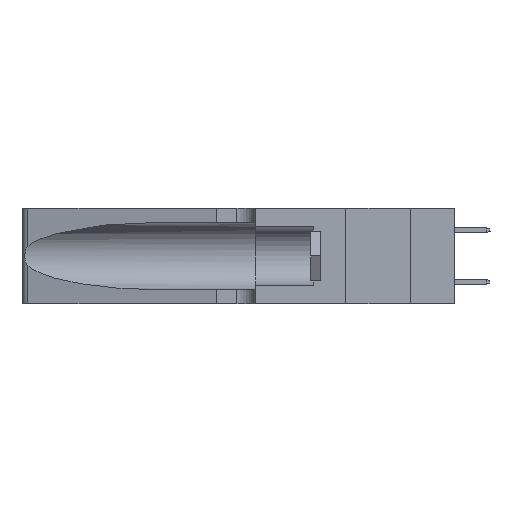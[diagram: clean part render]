
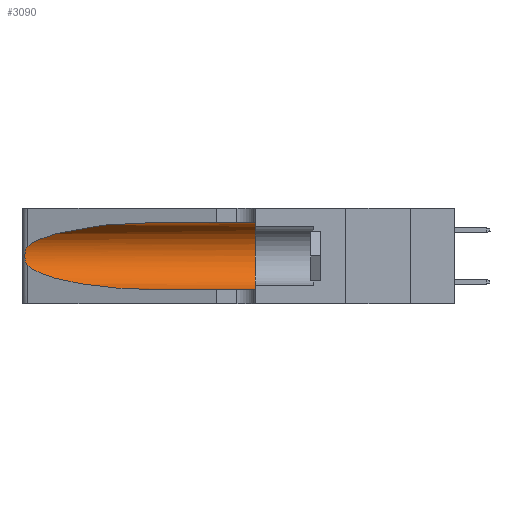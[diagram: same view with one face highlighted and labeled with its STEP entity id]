
A CAD part, left-side view. The second image highlights one B-rep face of the part: STEP entity #3090.
In plain terms, the highlighted cylindrical face has radius 3.308 mm (diameter 6.617 mm), a partial arc.
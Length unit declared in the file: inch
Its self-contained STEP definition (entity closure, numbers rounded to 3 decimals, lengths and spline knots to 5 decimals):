
#800 = VERTEX_POINT ( 'NONE', #20924 ) ;
#1029 = CARTESIAN_POINT ( 'NONE',  ( 0.25555, 1.22994, 0.2215 ) ) ;
#1853 = LINE ( 'NONE', #12380, #35251 ) ;
#2455 = EDGE_CURVE ( 'NONE', #5879, #4139, #14747, .T. ) ;
#2764 = EDGE_CURVE ( 'NONE', #34882, #5879, #6624, .T. ) ;
#3090 = ADVANCED_FACE ( 'NONE', ( #40278 ), #20788, .F. ) ;
#3096 = ORIENTED_EDGE ( 'NONE', *, *, #25256, .F. ) ;
#3694 = CARTESIAN_POINT ( 'NONE',  ( 0.25555, 1.22993, 0.14849 ) ) ;
#3937 = CARTESIAN_POINT ( 'NONE',  ( 0.25487, 1.22718, 0.22369 ) ) ;
#4139 = VERTEX_POINT ( 'NONE', #7296 ) ;
#5879 = VERTEX_POINT ( 'NONE', #3937 ) ;
#6624 =( BOUNDED_CURVE ( )  B_SPLINE_CURVE ( 3, ( #34306, #25080, #31236, #22221 ),
 .UNSPECIFIED., .F., .F. ) 
 B_SPLINE_CURVE_WITH_KNOTS ( ( 4, 4 ),
 ( 1.5708, 2.84003 ),
 .UNSPECIFIED. ) 
 CURVE ( )  GEOMETRIC_REPRESENTATION_ITEM ( )  RATIONAL_B_SPLINE_CURVE ( ( 1., 0.87, 0.87, 1. ) ) 
 REPRESENTATION_ITEM ( '' )  );
#7296 = CARTESIAN_POINT ( 'NONE',  ( 0.25487, 1.22718, 0.14631 ) ) ;
#7967 =( BOUNDED_CURVE ( )  B_SPLINE_CURVE ( 3, ( #25918, #32053, #32248, #25720 ),
 .UNSPECIFIED., .F., .F. ) 
 B_SPLINE_CURVE_WITH_KNOTS ( ( 4, 4 ),
 ( 3.44316, 4.71239 ),
 .UNSPECIFIED. ) 
 CURVE ( )  GEOMETRIC_REPRESENTATION_ITEM ( )  RATIONAL_B_SPLINE_CURVE ( ( 1., 0.87, 0.87, 1. ) ) 
 REPRESENTATION_ITEM ( '' )  );
#8767 = ORIENTED_EDGE ( 'NONE', *, *, #2455, .T. ) ;
#9604 = AXIS2_PLACEMENT_3D ( 'NONE', #17501, #29989, #11942 ) ;
#10426 = VERTEX_POINT ( 'NONE', #34806 ) ;
#10876 = CARTESIAN_POINT ( 'NONE',  ( 0.25639, 1.23184, 0.21858 ) ) ;
#11942 = DIRECTION ( 'NONE',  ( 0., 0., -1. ) ) ;
#12380 = CARTESIAN_POINT ( 'NONE',  ( 0.1305, 1.61858, 0.31525 ) ) ;
#12603 = CARTESIAN_POINT ( 'NONE',  ( 0.1305, 0.35, 0.185 ) ) ;
#12998 = VECTOR ( 'NONE', #23876, 39.37008 ) ;
#13142 = CARTESIAN_POINT ( 'NONE',  ( 0.25487, 1.22718, 0.14631 ) ) ;
#14747 = B_SPLINE_CURVE_WITH_KNOTS ( 'NONE', 3,
 ( #38996, #1029, #10876, #26059, #28700, #23003, #26262, #22585, #34860, #19287, #19499, #38593, #3694, #13142 ),
 .UNSPECIFIED., .F., .F.,
 ( 4, 2, 2, 2, 2, 2, 4 ),
 ( 0., 0.00027, 0.00053, 0.00107, 0.0016, 0.00187, 0.00214 ),
 .UNSPECIFIED. ) ;
#16407 = ORIENTED_EDGE ( 'NONE', *, *, #27896, .T. ) ;
#17395 = ORIENTED_EDGE ( 'NONE', *, *, #2764, .T. ) ;
#17501 = CARTESIAN_POINT ( 'NONE',  ( 0.1305, 1.61858, 0.185 ) ) ;
#19287 = CARTESIAN_POINT ( 'NONE',  ( 0.25856, 1.23593, 0.16098 ) ) ;
#19499 = CARTESIAN_POINT ( 'NONE',  ( 0.25789, 1.23486, 0.15765 ) ) ;
#20788 = CYLINDRICAL_SURFACE ( 'NONE', #9604, 0.13025 ) ;
#20924 = CARTESIAN_POINT ( 'NONE',  ( 0.1305, 0.35, 0.05475 ) ) ;
#20997 = CARTESIAN_POINT ( 'NONE',  ( 0.1305, 1.61858, 0.05475 ) ) ;
#21957 = CARTESIAN_POINT ( 'NONE',  ( 0.1305, 0.72297, 0.05475 ) ) ;
#22221 = CARTESIAN_POINT ( 'NONE',  ( 0.25487, 1.22718, 0.22369 ) ) ;
#22372 = EDGE_LOOP ( 'NONE', ( #17395, #8767, #38444, #16407, #3096, #34793 ) ) ;
#22585 = CARTESIAN_POINT ( 'NONE',  ( 0.26075, 1.23896, 0.178 ) ) ;
#23003 = CARTESIAN_POINT ( 'NONE',  ( 0.26018, 1.23835, 0.19895 ) ) ;
#23223 = VERTEX_POINT ( 'NONE', #21957 ) ;
#23876 = DIRECTION ( 'NONE',  ( 0., -1., 0. ) ) ;
#25080 = CARTESIAN_POINT ( 'NONE',  ( 0.18966, 0.96281, 0.31525 ) ) ;
#25106 = DIRECTION ( 'NONE',  ( 0., 0., 1. ) ) ;
#25256 = EDGE_CURVE ( 'NONE', #10426, #800, #37852, .T. ) ;
#25720 = CARTESIAN_POINT ( 'NONE',  ( 0.1305, 0.72297, 0.05475 ) ) ;
#25918 = CARTESIAN_POINT ( 'NONE',  ( 0.25487, 1.22718, 0.14631 ) ) ;
#26059 = CARTESIAN_POINT ( 'NONE',  ( 0.25787, 1.23484, 0.2124 ) ) ;
#26262 = CARTESIAN_POINT ( 'NONE',  ( 0.26075, 1.23896, 0.19203 ) ) ;
#27896 = EDGE_CURVE ( 'NONE', #23223, #800, #33887, .T. ) ;
#28012 = AXIS2_PLACEMENT_3D ( 'NONE', #12603, #31454, #25106 ) ;
#28170 = EDGE_CURVE ( 'NONE', #34882, #10426, #1853, .T. ) ;
#28700 = CARTESIAN_POINT ( 'NONE',  ( 0.25854, 1.2359, 0.20912 ) ) ;
#29989 = DIRECTION ( 'NONE',  ( 0., -1., 0. ) ) ;
#30869 = CARTESIAN_POINT ( 'NONE',  ( 0.1305, 0.72297, 0.31525 ) ) ;
#31236 = CARTESIAN_POINT ( 'NONE',  ( 0.2373, 1.15595, 0.28018 ) ) ;
#31454 = DIRECTION ( 'NONE',  ( 0., 1., 0. ) ) ;
#32053 = CARTESIAN_POINT ( 'NONE',  ( 0.2373, 1.15595, 0.08982 ) ) ;
#32248 = CARTESIAN_POINT ( 'NONE',  ( 0.18966, 0.96281, 0.05475 ) ) ;
#33733 = EDGE_CURVE ( 'NONE', #4139, #23223, #7967, .T. ) ;
#33887 = LINE ( 'NONE', #20997, #12998 ) ;
#34306 = CARTESIAN_POINT ( 'NONE',  ( 0.1305, 0.72297, 0.31525 ) ) ;
#34793 = ORIENTED_EDGE ( 'NONE', *, *, #28170, .F. ) ;
#34806 = CARTESIAN_POINT ( 'NONE',  ( 0.1305, 0.35, 0.31525 ) ) ;
#34860 = CARTESIAN_POINT ( 'NONE',  ( 0.26017, 1.23833, 0.17102 ) ) ;
#34882 = VERTEX_POINT ( 'NONE', #30869 ) ;
#35251 = VECTOR ( 'NONE', #37410, 39.37008 ) ;
#37410 = DIRECTION ( 'NONE',  ( 0., -1., 0. ) ) ;
#37852 = CIRCLE ( 'NONE', #28012, 0.13025 ) ;
#38444 = ORIENTED_EDGE ( 'NONE', *, *, #33733, .T. ) ;
#38593 = CARTESIAN_POINT ( 'NONE',  ( 0.25639, 1.23186, 0.15144 ) ) ;
#38996 = CARTESIAN_POINT ( 'NONE',  ( 0.25487, 1.22718, 0.22369 ) ) ;
#40278 = FACE_OUTER_BOUND ( 'NONE', #22372, .T. ) ;
